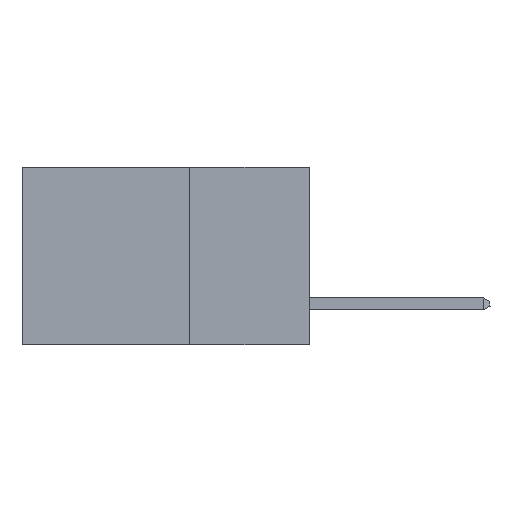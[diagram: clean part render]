
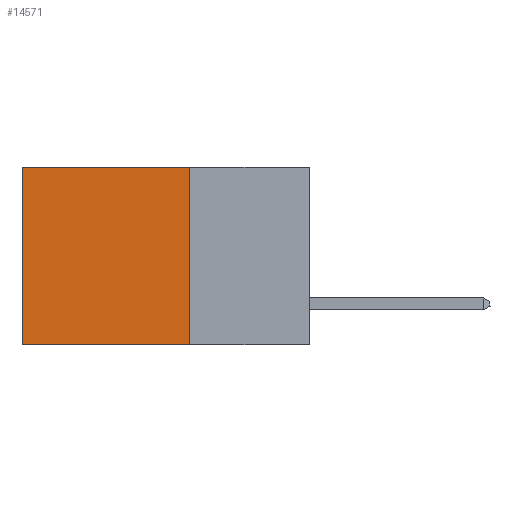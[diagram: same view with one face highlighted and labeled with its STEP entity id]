
A CAD part, left-side view. The second image highlights one B-rep face of the part: STEP entity #14571.
In plain terms, the highlighted planar face has unit normal (-1, 0, 0).
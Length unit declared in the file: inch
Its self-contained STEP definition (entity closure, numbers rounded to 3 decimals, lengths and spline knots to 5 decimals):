
#34 = CARTESIAN_POINT ( 'NONE',  ( 0.2875, 0.6, 0. ) ) ;
#314 = FACE_OUTER_BOUND ( 'NONE', #4865, .T. ) ;
#509 = VECTOR ( 'NONE', #1523, 39.37008 ) ;
#1496 = EDGE_CURVE ( 'NONE', #12176, #9495, #12387, .T. ) ;
#1523 = DIRECTION ( 'NONE',  ( 0., 0., -1. ) ) ;
#1713 = CARTESIAN_POINT ( 'NONE',  ( 0.2875, 0.6, 0. ) ) ;
#2051 = CARTESIAN_POINT ( 'NONE',  ( 0.2875, 0.6, -0.37 ) ) ;
#2681 = CARTESIAN_POINT ( 'NONE',  ( 0.2875, 0.25, 0. ) ) ;
#3877 = CARTESIAN_POINT ( 'NONE',  ( 0.2875, 0.25, 0. ) ) ;
#4443 = LINE ( 'NONE', #6471, #15067 ) ;
#4865 = EDGE_LOOP ( 'NONE', ( #11165, #18269, #7579, #9569 ) ) ;
#5093 = DIRECTION ( 'NONE',  ( 1., 0., 0. ) ) ;
#5771 = EDGE_CURVE ( 'NONE', #17478, #12176, #10151, .T. ) ;
#5907 = VECTOR ( 'NONE', #15740, 39.37008 ) ;
#6471 = CARTESIAN_POINT ( 'NONE',  ( 0.2875, 0.25, -0.37 ) ) ;
#7579 = ORIENTED_EDGE ( 'NONE', *, *, #11827, .F. ) ;
#7922 = CARTESIAN_POINT ( 'NONE',  ( 0.2875, 0.25, 0. ) ) ;
#8346 = CARTESIAN_POINT ( 'NONE',  ( 0.2875, 0.25, 0. ) ) ;
#9495 = VERTEX_POINT ( 'NONE', #2051 ) ;
#9569 = ORIENTED_EDGE ( 'NONE', *, *, #5771, .T. ) ;
#10151 = LINE ( 'NONE', #7922, #13577 ) ;
#11054 = DIRECTION ( 'NONE',  ( 0., 0., -1. ) ) ;
#11165 = ORIENTED_EDGE ( 'NONE', *, *, #1496, .T. ) ;
#11827 = EDGE_CURVE ( 'NONE', #17478, #16758, #13741, .T. ) ;
#12176 = VERTEX_POINT ( 'NONE', #1713 ) ;
#12387 = LINE ( 'NONE', #34, #509 ) ;
#12557 = AXIS2_PLACEMENT_3D ( 'NONE', #8346, #5093, #11054 ) ;
#13239 = EDGE_CURVE ( 'NONE', #16758, #9495, #4443, .T. ) ;
#13577 = VECTOR ( 'NONE', #13667, 39.37008 ) ;
#13667 = DIRECTION ( 'NONE',  ( 0., 1., 0. ) ) ;
#13741 = LINE ( 'NONE', #3877, #5907 ) ;
#13879 = DIRECTION ( 'NONE',  ( 0., 1., 0. ) ) ;
#14571 = ADVANCED_FACE ( 'NONE', ( #314 ), #15439, .F. ) ;
#15067 = VECTOR ( 'NONE', #13879, 39.37008 ) ;
#15439 = PLANE ( 'NONE',  #12557 ) ;
#15740 = DIRECTION ( 'NONE',  ( 0., 0., -1. ) ) ;
#15748 = CARTESIAN_POINT ( 'NONE',  ( 0.2875, 0.25, -0.37 ) ) ;
#16758 = VERTEX_POINT ( 'NONE', #15748 ) ;
#17478 = VERTEX_POINT ( 'NONE', #2681 ) ;
#18269 = ORIENTED_EDGE ( 'NONE', *, *, #13239, .F. ) ;
